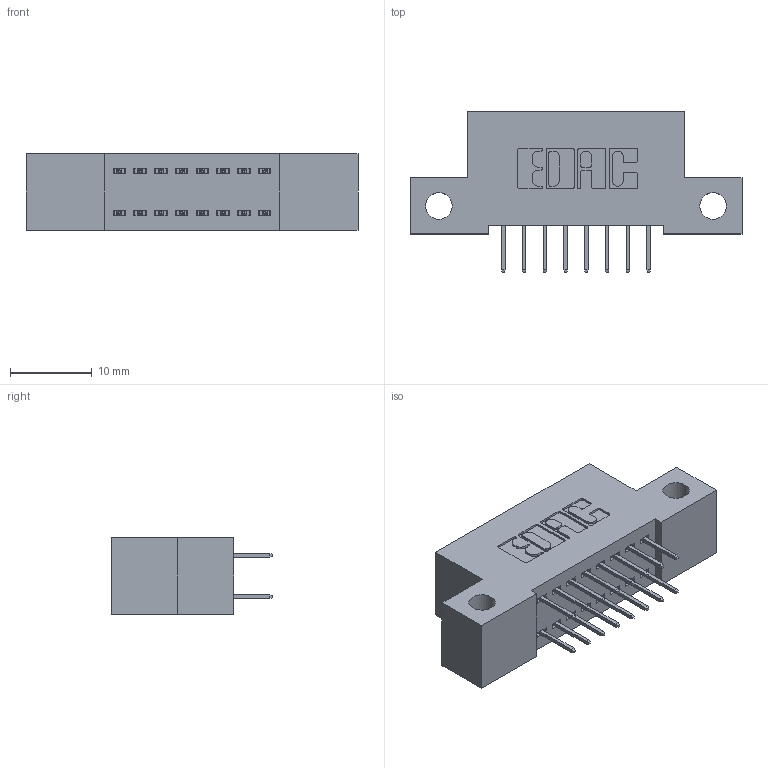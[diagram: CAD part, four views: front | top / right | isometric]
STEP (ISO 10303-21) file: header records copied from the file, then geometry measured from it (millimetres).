
FILE_DESCRIPTION (( 'STEP AP203' ), '1' );
FILE_NAME ('342-016-524-212.STEP', '2019-10-01T18:49:47', ( '' ), ( '' ), 'SwSTEP 2.0', 'SolidWorks 2016', '' );
FILE_SCHEMA (( 'CONFIG_CONTROL_DESIGN' ));
Length unit declared in the file: inch
Products named in the file (3): 342-016-524-212; 342 Part_Side Mount; 345-292-001_345-293-124
Assembly tree (17 placements, depth 2):
  342-016-524-212
    342 Part_Side Mount
    345-292-001_345-293-124  x16
Bounding box: 40.64 x 19.69 x 9.4 mm (x, y, z)
Volume: 3392.4 mm3; surface area: 4461.5 mm2
Topology: 17 solids, 17 shells, 1006 faces, 2843 edges, 1830 vertices
Faces by surface type: plane 738, cylinder 268
Entity records: 9489 total; most frequent: CARTESIAN_POINT 1610, ORIENTED_EDGE 1546, DIRECTION 1437, EDGE_CURVE 773, VECTOR 649, LINE 649, VERTEX_POINT 510, AXIS2_PLACEMENT_3D 394
